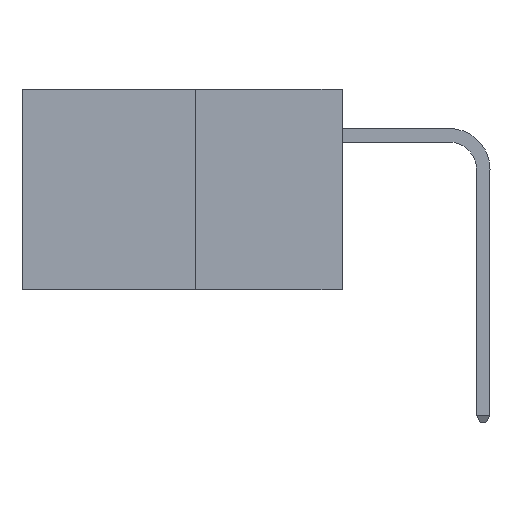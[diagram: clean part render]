
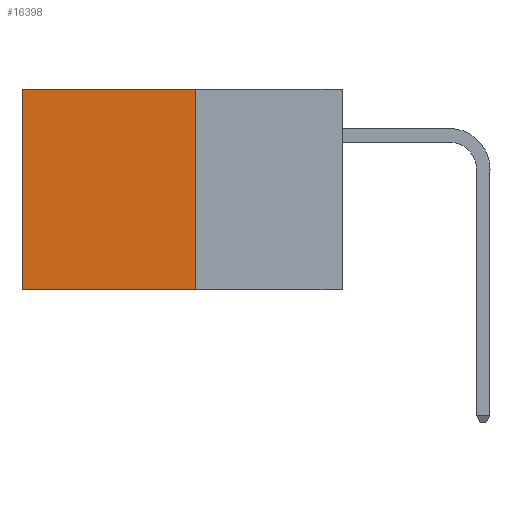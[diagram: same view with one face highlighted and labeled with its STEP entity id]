
A CAD part, left-side view. The second image highlights one B-rep face of the part: STEP entity #16398.
In plain terms, the highlighted planar face has unit normal (-1, 0, 0).
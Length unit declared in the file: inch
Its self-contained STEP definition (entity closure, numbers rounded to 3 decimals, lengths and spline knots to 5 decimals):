
#358 = VERTEX_POINT ( 'NONE', #17997 ) ;
#375 = VECTOR ( 'NONE', #9092, 39.37008 ) ;
#400 = AXIS2_PLACEMENT_3D ( 'NONE', #19079, #20829, #10142 ) ;
#2151 = LINE ( 'NONE', #8838, #375 ) ;
#3085 = EDGE_CURVE ( 'NONE', #358, #11687, #2151, .T. ) ;
#4249 = ORIENTED_EDGE ( 'NONE', *, *, #3085, .T. ) ;
#5368 = VERTEX_POINT ( 'NONE', #8571 ) ;
#6416 = PLANE ( 'NONE',  #400 ) ;
#6643 = LINE ( 'NONE', #8066, #10405 ) ;
#6906 = VECTOR ( 'NONE', #22208, 39.37008 ) ;
#7618 = EDGE_LOOP ( 'NONE', ( #10818, #21072, #8918, #4249 ) ) ;
#7619 = VECTOR ( 'NONE', #8712, 39.37008 ) ;
#7890 = CARTESIAN_POINT ( 'NONE',  ( 0.277, 0.27, -0.37 ) ) ;
#8066 = CARTESIAN_POINT ( 'NONE',  ( 0.277, 0.27, -0.37 ) ) ;
#8571 = CARTESIAN_POINT ( 'NONE',  ( 0.277, 0.59, -0.37 ) ) ;
#8712 = DIRECTION ( 'NONE',  ( 0., 0., -1. ) ) ;
#8838 = CARTESIAN_POINT ( 'NONE',  ( 0.277, 0.27, 0. ) ) ;
#8918 = ORIENTED_EDGE ( 'NONE', *, *, #11484, .F. ) ;
#9092 = DIRECTION ( 'NONE',  ( 0., 1., 0. ) ) ;
#10142 = DIRECTION ( 'NONE',  ( 0., 0., -1. ) ) ;
#10405 = VECTOR ( 'NONE', #15356, 39.37008 ) ;
#10592 = CARTESIAN_POINT ( 'NONE',  ( 0.277, 0.59, -0.37 ) ) ;
#10616 = CARTESIAN_POINT ( 'NONE',  ( 0.277, 0.59, 0. ) ) ;
#10818 = ORIENTED_EDGE ( 'NONE', *, *, #12352, .T. ) ;
#10891 = EDGE_CURVE ( 'NONE', #18657, #5368, #6643, .T. ) ;
#11484 = EDGE_CURVE ( 'NONE', #358, #18657, #21254, .T. ) ;
#11687 = VERTEX_POINT ( 'NONE', #10616 ) ;
#12352 = EDGE_CURVE ( 'NONE', #11687, #5368, #17800, .T. ) ;
#15356 = DIRECTION ( 'NONE',  ( 0., 1., 0. ) ) ;
#16398 = ADVANCED_FACE ( 'NONE', ( #21628 ), #6416, .F. ) ;
#17800 = LINE ( 'NONE', #10592, #7619 ) ;
#17997 = CARTESIAN_POINT ( 'NONE',  ( 0.277, 0.27, 0. ) ) ;
#18657 = VERTEX_POINT ( 'NONE', #21427 ) ;
#19079 = CARTESIAN_POINT ( 'NONE',  ( 0.277, 0.27, -0.37 ) ) ;
#20829 = DIRECTION ( 'NONE',  ( 1., 0., 0. ) ) ;
#21072 = ORIENTED_EDGE ( 'NONE', *, *, #10891, .F. ) ;
#21254 = LINE ( 'NONE', #7890, #6906 ) ;
#21427 = CARTESIAN_POINT ( 'NONE',  ( 0.277, 0.27, -0.37 ) ) ;
#21628 = FACE_OUTER_BOUND ( 'NONE', #7618, .T. ) ;
#22208 = DIRECTION ( 'NONE',  ( 0., 0., -1. ) ) ;
